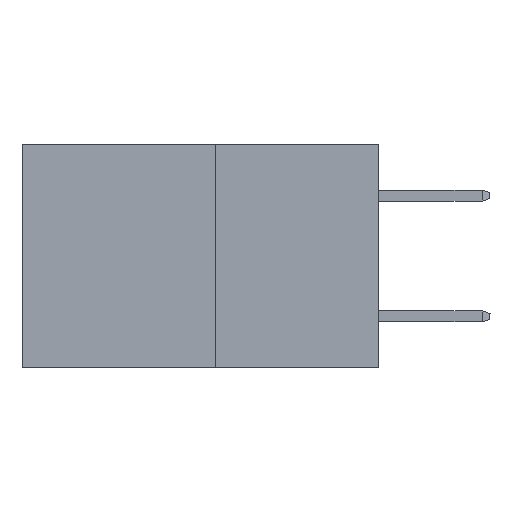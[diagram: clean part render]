
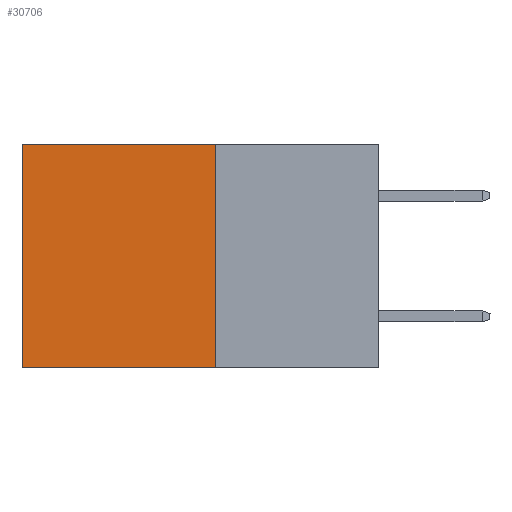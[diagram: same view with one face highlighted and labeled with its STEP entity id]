
A CAD part, left-side view. The second image highlights one B-rep face of the part: STEP entity #30706.
In plain terms, the highlighted planar face has unit normal (-1, 0, 0).
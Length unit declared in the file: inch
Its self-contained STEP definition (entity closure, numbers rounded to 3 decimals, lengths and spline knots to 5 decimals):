
#170 = LINE ( 'NONE', #5855, #28001 ) ;
#1603 = ORIENTED_EDGE ( 'NONE', *, *, #32936, .F. ) ;
#4076 = VECTOR ( 'NONE', #16506, 39.37008 ) ;
#4431 = CARTESIAN_POINT ( 'NONE',  ( 0.277, 0.27, -0.37 ) ) ;
#4823 = VECTOR ( 'NONE', #12703, 39.37008 ) ;
#4938 = LINE ( 'NONE', #13709, #4076 ) ;
#5855 = CARTESIAN_POINT ( 'NONE',  ( 0.277, 0.27, -0.37 ) ) ;
#6169 = EDGE_CURVE ( 'NONE', #23449, #16395, #170, .T. ) ;
#10047 = DIRECTION ( 'NONE',  ( 0., 0., -1. ) ) ;
#12679 = CARTESIAN_POINT ( 'NONE',  ( 0.277, 0.59, -0.37 ) ) ;
#12703 = DIRECTION ( 'NONE',  ( 0., 0., -1. ) ) ;
#13188 = VERTEX_POINT ( 'NONE', #15519 ) ;
#13235 = CARTESIAN_POINT ( 'NONE',  ( 0.277, 0.27, -0.37 ) ) ;
#13350 = DIRECTION ( 'NONE',  ( 0., 0., -1. ) ) ;
#13709 = CARTESIAN_POINT ( 'NONE',  ( 0.277, 0.27, 0. ) ) ;
#14121 = LINE ( 'NONE', #12679, #27983 ) ;
#15494 = ORIENTED_EDGE ( 'NONE', *, *, #16466, .T. ) ;
#15519 = CARTESIAN_POINT ( 'NONE',  ( 0.277, 0.27, 0. ) ) ;
#15810 = ORIENTED_EDGE ( 'NONE', *, *, #17425, .T. ) ;
#16345 = VERTEX_POINT ( 'NONE', #31284 ) ;
#16395 = VERTEX_POINT ( 'NONE', #28940 ) ;
#16466 = EDGE_CURVE ( 'NONE', #16345, #16395, #14121, .T. ) ;
#16506 = DIRECTION ( 'NONE',  ( 0., 1., 0. ) ) ;
#17425 = EDGE_CURVE ( 'NONE', #13188, #16345, #4938, .T. ) ;
#20020 = ORIENTED_EDGE ( 'NONE', *, *, #6169, .F. ) ;
#20956 = AXIS2_PLACEMENT_3D ( 'NONE', #13235, #29930, #13350 ) ;
#22440 = DIRECTION ( 'NONE',  ( 0., 1., 0. ) ) ;
#23449 = VERTEX_POINT ( 'NONE', #4431 ) ;
#26525 = CARTESIAN_POINT ( 'NONE',  ( 0.277, 0.27, -0.37 ) ) ;
#26898 = EDGE_LOOP ( 'NONE', ( #15494, #20020, #1603, #15810 ) ) ;
#27125 = PLANE ( 'NONE',  #20956 ) ;
#27983 = VECTOR ( 'NONE', #10047, 39.37008 ) ;
#28001 = VECTOR ( 'NONE', #22440, 39.37008 ) ;
#28940 = CARTESIAN_POINT ( 'NONE',  ( 0.277, 0.59, -0.37 ) ) ;
#29930 = DIRECTION ( 'NONE',  ( 1., 0., 0. ) ) ;
#30706 = ADVANCED_FACE ( 'NONE', ( #35233 ), #27125, .F. ) ;
#31284 = CARTESIAN_POINT ( 'NONE',  ( 0.277, 0.59, 0. ) ) ;
#32936 = EDGE_CURVE ( 'NONE', #13188, #23449, #34203, .T. ) ;
#34203 = LINE ( 'NONE', #26525, #4823 ) ;
#35233 = FACE_OUTER_BOUND ( 'NONE', #26898, .T. ) ;
